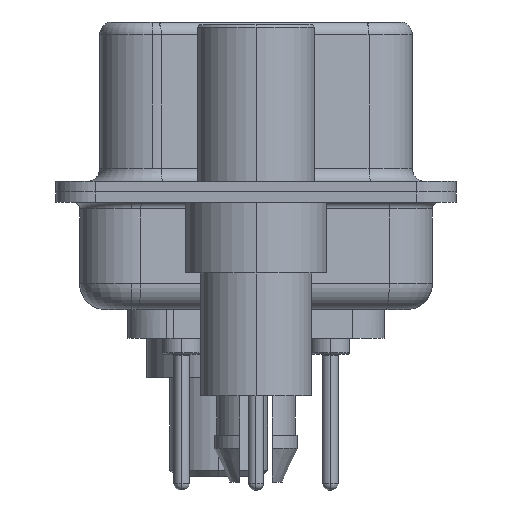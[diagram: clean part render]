
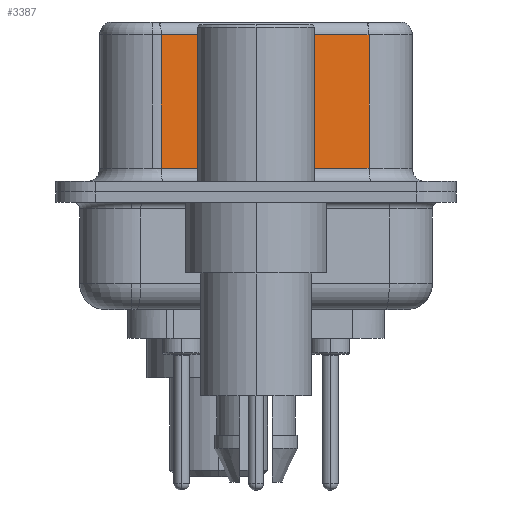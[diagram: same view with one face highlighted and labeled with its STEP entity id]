
A CAD part, left-side view. The second image highlights one B-rep face of the part: STEP entity #3387.
In plain terms, the highlighted planar face has unit normal (-0.985, -0.174, 0).
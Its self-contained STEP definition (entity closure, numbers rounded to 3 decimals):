
#2369 = EDGE_CURVE ( 'NONE', #21606, #24645, #28412, .T. ) ;
#2475 = VERTEX_POINT ( 'NONE', #26615 ) ;
#3387 = ADVANCED_FACE ( 'NONE', ( #8345 ), #26658, .F. ) ;
#3434 = EDGE_LOOP ( 'NONE', ( #14492, #27629, #19819, #13563 ) ) ;
#4265 = DIRECTION ( 'NONE',  ( 0., 0., -1. ) ) ;
#5155 = CARTESIAN_POINT ( 'NONE',  ( 3.73, 3.628, 6.52 ) ) ;
#5912 = VERTEX_POINT ( 'NONE', #8795 ) ;
#6330 = EDGE_CURVE ( 'NONE', #21606, #2475, #27578, .T. ) ;
#7016 = VECTOR ( 'NONE', #4265, 1000. ) ;
#7425 = DIRECTION ( 'NONE',  ( 0., 0., -1. ) ) ;
#8345 = FACE_OUTER_BOUND ( 'NONE', #3434, .T. ) ;
#8795 = CARTESIAN_POINT ( 'NONE',  ( 3.73, 3.628, 0.9 ) ) ;
#8871 = CARTESIAN_POINT ( 'NONE',  ( 5.132, -4.322, 6.02 ) ) ;
#9249 = CARTESIAN_POINT ( 'NONE',  ( 5.132, -4.322, 0.9 ) ) ;
#9792 = LINE ( 'NONE', #5155, #22222 ) ;
#10206 = DIRECTION ( 'NONE',  ( -0.174, 0.985, 0. ) ) ;
#10712 = LINE ( 'NONE', #24566, #16594 ) ;
#13563 = ORIENTED_EDGE ( 'NONE', *, *, #21662, .T. ) ;
#13566 = DIRECTION ( 'NONE',  ( 0.174, -0.985, 0. ) ) ;
#14492 = ORIENTED_EDGE ( 'NONE', *, *, #2369, .F. ) ;
#16594 = VECTOR ( 'NONE', #13566, 1000. ) ;
#19288 = DIRECTION ( 'NONE',  ( 0.985, 0.174, 0. ) ) ;
#19747 = CARTESIAN_POINT ( 'NONE',  ( 5.132, -4.322, 6.52 ) ) ;
#19819 = ORIENTED_EDGE ( 'NONE', *, *, #26961, .T. ) ;
#21606 = VERTEX_POINT ( 'NONE', #8871 ) ;
#21662 = EDGE_CURVE ( 'NONE', #5912, #24645, #10712, .T. ) ;
#21696 = VECTOR ( 'NONE', #10206, 1000. ) ;
#22083 = DIRECTION ( 'NONE',  ( -0.174, 0.985, 0. ) ) ;
#22222 = VECTOR ( 'NONE', #7425, 1000. ) ;
#22587 = AXIS2_PLACEMENT_3D ( 'NONE', #28321, #19288, #22083 ) ;
#24566 = CARTESIAN_POINT ( 'NONE',  ( 5.132, -4.322, 0.9 ) ) ;
#24645 = VERTEX_POINT ( 'NONE', #9249 ) ;
#25411 = CARTESIAN_POINT ( 'NONE',  ( 5.132, -4.322, 6.02 ) ) ;
#26615 = CARTESIAN_POINT ( 'NONE',  ( 3.73, 3.628, 6.02 ) ) ;
#26658 = PLANE ( 'NONE',  #22587 ) ;
#26961 = EDGE_CURVE ( 'NONE', #2475, #5912, #9792, .T. ) ;
#27578 = LINE ( 'NONE', #25411, #21696 ) ;
#27629 = ORIENTED_EDGE ( 'NONE', *, *, #6330, .T. ) ;
#28321 = CARTESIAN_POINT ( 'NONE',  ( 5.132, -4.322, 6.52 ) ) ;
#28412 = LINE ( 'NONE', #19747, #7016 ) ;
